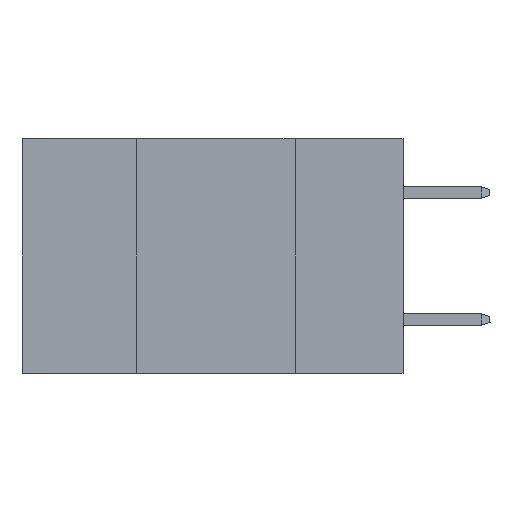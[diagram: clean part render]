
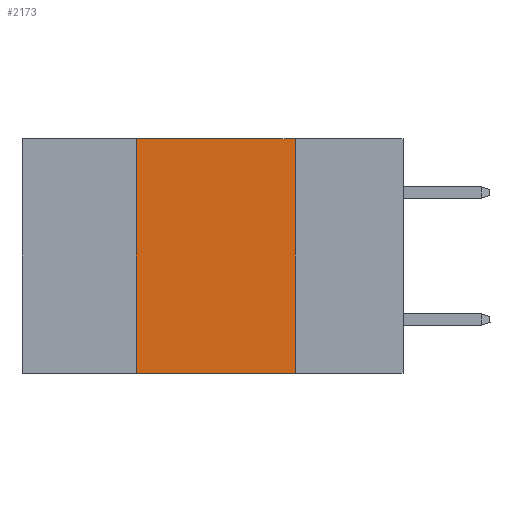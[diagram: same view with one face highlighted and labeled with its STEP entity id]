
A CAD part, left-side view. The second image highlights one B-rep face of the part: STEP entity #2173.
In plain terms, the highlighted planar face has unit normal (-1, 0, 0).
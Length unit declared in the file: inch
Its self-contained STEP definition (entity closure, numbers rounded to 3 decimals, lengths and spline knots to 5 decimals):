
#546 = EDGE_CURVE ( 'NONE', #23798, #8868, #9825, .T. ) ;
#920 = DIRECTION ( 'NONE',  ( 0., 0., 1. ) ) ;
#1827 = PLANE ( 'NONE',  #14157 ) ;
#2173 = ADVANCED_FACE ( 'NONE', ( #9858 ), #1827, .F. ) ;
#2367 = CARTESIAN_POINT ( 'NONE',  ( 0., 0.42, 0. ) ) ;
#3728 = DIRECTION ( 'NONE',  ( 0., -1., 0. ) ) ;
#3796 = DIRECTION ( 'NONE',  ( 0., 0., -1. ) ) ;
#4774 = VECTOR ( 'NONE', #920, 39.37008 ) ;
#4827 = LINE ( 'NONE', #26390, #4774 ) ;
#6051 = VECTOR ( 'NONE', #12988, 39.37008 ) ;
#7208 = ORIENTED_EDGE ( 'NONE', *, *, #24413, .F. ) ;
#7872 = LINE ( 'NONE', #26685, #12695 ) ;
#7933 = EDGE_LOOP ( 'NONE', ( #13383, #25545, #7208, #8802 ) ) ;
#8802 = ORIENTED_EDGE ( 'NONE', *, *, #546, .T. ) ;
#8868 = VERTEX_POINT ( 'NONE', #11409 ) ;
#9501 = CARTESIAN_POINT ( 'NONE',  ( 0., 0.17, 0. ) ) ;
#9825 = LINE ( 'NONE', #11516, #25851 ) ;
#9858 = FACE_OUTER_BOUND ( 'NONE', #7933, .T. ) ;
#11073 = EDGE_CURVE ( 'NONE', #15751, #24367, #7872, .T. ) ;
#11409 = CARTESIAN_POINT ( 'NONE',  ( 0., 0.17, -0.37 ) ) ;
#11516 = CARTESIAN_POINT ( 'NONE',  ( 0., 0.6, -0.37 ) ) ;
#12695 = VECTOR ( 'NONE', #3728, 39.37008 ) ;
#12988 = DIRECTION ( 'NONE',  ( 0., 0., -1. ) ) ;
#13383 = ORIENTED_EDGE ( 'NONE', *, *, #26749, .F. ) ;
#13853 = DIRECTION ( 'NONE',  ( 0., -1., 0. ) ) ;
#14157 = AXIS2_PLACEMENT_3D ( 'NONE', #18306, #26748, #3796 ) ;
#15057 = LINE ( 'NONE', #27230, #6051 ) ;
#15751 = VERTEX_POINT ( 'NONE', #2367 ) ;
#17424 = CARTESIAN_POINT ( 'NONE',  ( 0., 0.42, -0.37 ) ) ;
#18306 = CARTESIAN_POINT ( 'NONE',  ( 0., 0.6, 0. ) ) ;
#23798 = VERTEX_POINT ( 'NONE', #17424 ) ;
#24367 = VERTEX_POINT ( 'NONE', #9501 ) ;
#24413 = EDGE_CURVE ( 'NONE', #23798, #15751, #4827, .T. ) ;
#25545 = ORIENTED_EDGE ( 'NONE', *, *, #11073, .F. ) ;
#25851 = VECTOR ( 'NONE', #13853, 39.37008 ) ;
#26390 = CARTESIAN_POINT ( 'NONE',  ( 0., 0.42, 0. ) ) ;
#26685 = CARTESIAN_POINT ( 'NONE',  ( 0., 0.6, 0. ) ) ;
#26748 = DIRECTION ( 'NONE',  ( 1., 0., 0. ) ) ;
#26749 = EDGE_CURVE ( 'NONE', #24367, #8868, #15057, .T. ) ;
#27230 = CARTESIAN_POINT ( 'NONE',  ( 0., 0.17, 0. ) ) ;
